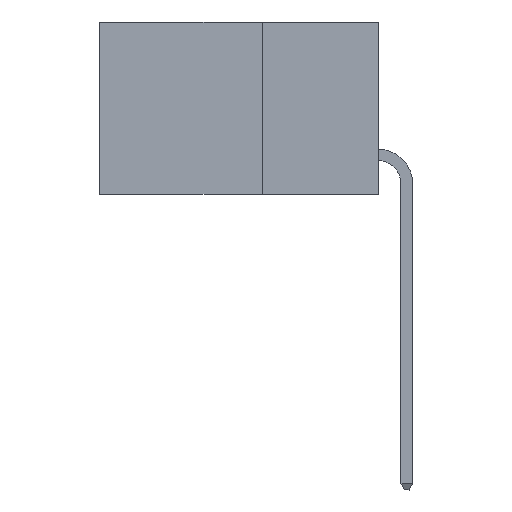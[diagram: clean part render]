
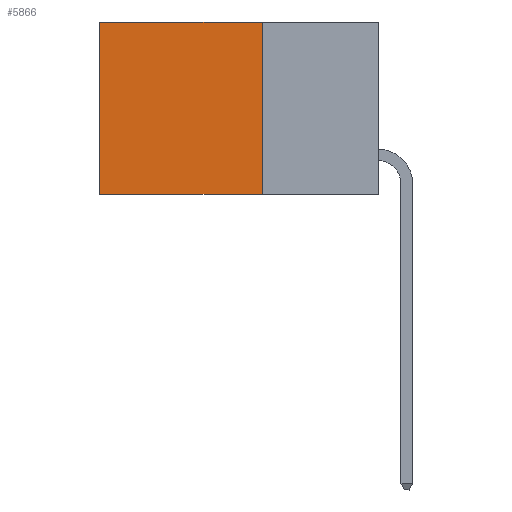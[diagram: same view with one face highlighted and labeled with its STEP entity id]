
A CAD part, left-side view. The second image highlights one B-rep face of the part: STEP entity #5866.
In plain terms, the highlighted planar face has unit normal (-1, 0, 0).
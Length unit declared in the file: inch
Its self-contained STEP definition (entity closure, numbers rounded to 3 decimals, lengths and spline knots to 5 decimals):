
#1056 = DIRECTION ( 'NONE',  ( 0., 0., -1. ) ) ;
#1514 = DIRECTION ( 'NONE',  ( 1., 0., 0. ) ) ;
#2110 = LINE ( 'NONE', #26028, #18166 ) ;
#4347 = LINE ( 'NONE', #20585, #25823 ) ;
#4570 = EDGE_CURVE ( 'NONE', #14932, #22392, #8904, .T. ) ;
#5471 = VERTEX_POINT ( 'NONE', #24955 ) ;
#5534 = DIRECTION ( 'NONE',  ( 0., 1., 0. ) ) ;
#5866 = ADVANCED_FACE ( 'NONE', ( #8827 ), #19827, .F. ) ;
#7127 = CARTESIAN_POINT ( 'NONE',  ( 0.298, 0.25, -0.37 ) ) ;
#8255 = EDGE_CURVE ( 'NONE', #5471, #22392, #2110, .T. ) ;
#8827 = FACE_OUTER_BOUND ( 'NONE', #16304, .T. ) ;
#8904 = LINE ( 'NONE', #12560, #14434 ) ;
#11193 = VECTOR ( 'NONE', #12744, 39.37008 ) ;
#12560 = CARTESIAN_POINT ( 'NONE',  ( 0.298, 0.25, -0.37 ) ) ;
#12587 = EDGE_CURVE ( 'NONE', #13216, #5471, #22278, .T. ) ;
#12744 = DIRECTION ( 'NONE',  ( 0., 1., 0. ) ) ;
#13216 = VERTEX_POINT ( 'NONE', #14546 ) ;
#14049 = CARTESIAN_POINT ( 'NONE',  ( 0.298, 0.25, 0. ) ) ;
#14272 = DIRECTION ( 'NONE',  ( 0., 0., -1. ) ) ;
#14434 = VECTOR ( 'NONE', #5534, 39.37008 ) ;
#14546 = CARTESIAN_POINT ( 'NONE',  ( 0.298, 0.25, 0. ) ) ;
#14932 = VERTEX_POINT ( 'NONE', #7127 ) ;
#15936 = EDGE_CURVE ( 'NONE', #13216, #14932, #4347, .T. ) ;
#16173 = DIRECTION ( 'NONE',  ( 0., 0., -1. ) ) ;
#16245 = ORIENTED_EDGE ( 'NONE', *, *, #15936, .F. ) ;
#16304 = EDGE_LOOP ( 'NONE', ( #16394, #18536, #16245, #18185 ) ) ;
#16394 = ORIENTED_EDGE ( 'NONE', *, *, #8255, .T. ) ;
#16978 = CARTESIAN_POINT ( 'NONE',  ( 0.298, 0.25, 0. ) ) ;
#17163 = CARTESIAN_POINT ( 'NONE',  ( 0.298, 0.6, -0.37 ) ) ;
#18166 = VECTOR ( 'NONE', #1056, 39.37008 ) ;
#18185 = ORIENTED_EDGE ( 'NONE', *, *, #12587, .T. ) ;
#18536 = ORIENTED_EDGE ( 'NONE', *, *, #4570, .F. ) ;
#19827 = PLANE ( 'NONE',  #23063 ) ;
#20585 = CARTESIAN_POINT ( 'NONE',  ( 0.298, 0.25, 0. ) ) ;
#22278 = LINE ( 'NONE', #16978, #11193 ) ;
#22392 = VERTEX_POINT ( 'NONE', #17163 ) ;
#23063 = AXIS2_PLACEMENT_3D ( 'NONE', #14049, #1514, #16173 ) ;
#24955 = CARTESIAN_POINT ( 'NONE',  ( 0.298, 0.6, 0. ) ) ;
#25823 = VECTOR ( 'NONE', #14272, 39.37008 ) ;
#26028 = CARTESIAN_POINT ( 'NONE',  ( 0.298, 0.6, 0. ) ) ;
